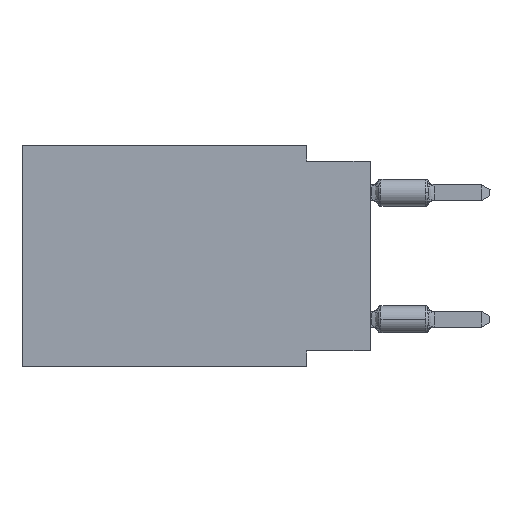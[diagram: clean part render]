
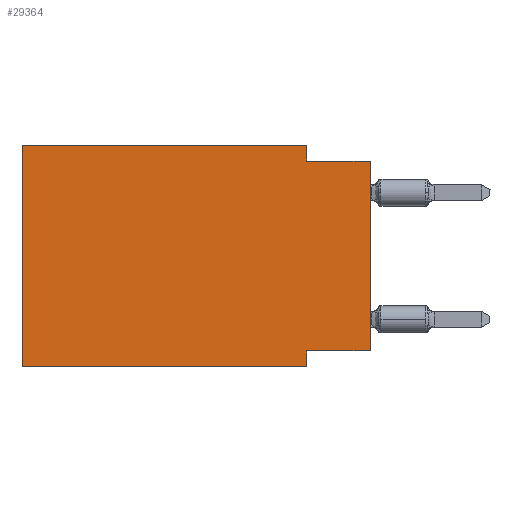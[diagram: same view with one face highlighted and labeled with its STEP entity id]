
A CAD part, left-side view. The second image highlights one B-rep face of the part: STEP entity #29364.
In plain terms, the highlighted planar face has unit normal (-1, 0, 0).
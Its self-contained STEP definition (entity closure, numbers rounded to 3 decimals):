
#2021 = DIRECTION ( 'NONE',  ( 0., -1., 0. ) ) ;
#2461 = CARTESIAN_POINT ( 'NONE',  ( 0., 0., -0.635 ) ) ;
#3961 = LINE ( 'NONE', #53313, #49097 ) ;
#5536 = DIRECTION ( 'NONE',  ( 0., 1., 0. ) ) ;
#6304 = CARTESIAN_POINT ( 'NONE',  ( 0., 13.97, 0. ) ) ;
#8507 = CARTESIAN_POINT ( 'NONE',  ( 0., 0., -8.255 ) ) ;
#9476 = CARTESIAN_POINT ( 'NONE',  ( 0., 0., -8.255 ) ) ;
#12261 = VERTEX_POINT ( 'NONE', #36278 ) ;
#12854 = LINE ( 'NONE', #33923, #29108 ) ;
#14314 = CARTESIAN_POINT ( 'NONE',  ( 0., 13.97, -8.89 ) ) ;
#15795 = ORIENTED_EDGE ( 'NONE', *, *, #59876, .F. ) ;
#16778 = VERTEX_POINT ( 'NONE', #42042 ) ;
#18086 = CARTESIAN_POINT ( 'NONE',  ( 0., 2.54, 0. ) ) ;
#18163 = EDGE_CURVE ( 'NONE', #12261, #36258, #45525, .T. ) ;
#18897 = DIRECTION ( 'NONE',  ( 0., 0., -1. ) ) ;
#21509 = CARTESIAN_POINT ( 'NONE',  ( 0., 0., -0.635 ) ) ;
#22657 = ORIENTED_EDGE ( 'NONE', *, *, #27239, .F. ) ;
#24183 = DIRECTION ( 'NONE',  ( 1., 0., 0. ) ) ;
#25414 = VECTOR ( 'NONE', #57253, 1000. ) ;
#25524 = VECTOR ( 'NONE', #40719, 1000. ) ;
#25767 = EDGE_LOOP ( 'NONE', ( #29877, #28034, #40921, #15795, #50208, #28867, #22657, #38888 ) ) ;
#27239 = EDGE_CURVE ( 'NONE', #38077, #16778, #3961, .T. ) ;
#27383 = LINE ( 'NONE', #27701, #25414 ) ;
#27456 = VERTEX_POINT ( 'NONE', #14314 ) ;
#27701 = CARTESIAN_POINT ( 'NONE',  ( 0., 13.97, -8.89 ) ) ;
#28034 = ORIENTED_EDGE ( 'NONE', *, *, #18163, .F. ) ;
#28680 = VERTEX_POINT ( 'NONE', #43931 ) ;
#28867 = ORIENTED_EDGE ( 'NONE', *, *, #59912, .T. ) ;
#29108 = VECTOR ( 'NONE', #33284, 1000. ) ;
#29364 = ADVANCED_FACE ( 'NONE', ( #64038 ), #59511, .F. ) ;
#29877 = ORIENTED_EDGE ( 'NONE', *, *, #52129, .T. ) ;
#33284 = DIRECTION ( 'NONE',  ( 0., 0., -1. ) ) ;
#33923 = CARTESIAN_POINT ( 'NONE',  ( 0., 2.54, 0. ) ) ;
#34381 = VECTOR ( 'NONE', #2021, 1000. ) ;
#35752 = DIRECTION ( 'NONE',  ( 0., 0., 1. ) ) ;
#35804 = VECTOR ( 'NONE', #60803, 1000. ) ;
#36258 = VERTEX_POINT ( 'NONE', #2461 ) ;
#36278 = CARTESIAN_POINT ( 'NONE',  ( 0., 2.54, -0.635 ) ) ;
#36370 = CARTESIAN_POINT ( 'NONE',  ( 0., 0., 0. ) ) ;
#38077 = VERTEX_POINT ( 'NONE', #58702 ) ;
#38294 = VERTEX_POINT ( 'NONE', #18086 ) ;
#38804 = DIRECTION ( 'NONE',  ( 0., 0., -1. ) ) ;
#38888 = ORIENTED_EDGE ( 'NONE', *, *, #45697, .F. ) ;
#38896 = EDGE_CURVE ( 'NONE', #27456, #28680, #60504, .T. ) ;
#40719 = DIRECTION ( 'NONE',  ( 0., 0., 1. ) ) ;
#40921 = ORIENTED_EDGE ( 'NONE', *, *, #47215, .F. ) ;
#41686 = VECTOR ( 'NONE', #5536, 1000. ) ;
#42042 = CARTESIAN_POINT ( 'NONE',  ( 0., 2.54, -8.89 ) ) ;
#43931 = CARTESIAN_POINT ( 'NONE',  ( 0., 13.97, 0. ) ) ;
#44278 = CARTESIAN_POINT ( 'NONE',  ( 0., 13.97, 0. ) ) ;
#44645 = VECTOR ( 'NONE', #35752, 1000. ) ;
#45525 = LINE ( 'NONE', #21509, #34381 ) ;
#45697 = EDGE_CURVE ( 'NONE', #55185, #38077, #54858, .T. ) ;
#47215 = EDGE_CURVE ( 'NONE', #38294, #12261, #12854, .T. ) ;
#49097 = VECTOR ( 'NONE', #18897, 1000. ) ;
#49463 = AXIS2_PLACEMENT_3D ( 'NONE', #44278, #24183, #38804 ) ;
#50208 = ORIENTED_EDGE ( 'NONE', *, *, #38896, .F. ) ;
#52129 = EDGE_CURVE ( 'NONE', #55185, #36258, #55211, .T. ) ;
#53313 = CARTESIAN_POINT ( 'NONE',  ( 0., 2.54, -8.89 ) ) ;
#54858 = LINE ( 'NONE', #9476, #41686 ) ;
#54982 = LINE ( 'NONE', #6304, #35804 ) ;
#55185 = VERTEX_POINT ( 'NONE', #8507 ) ;
#55211 = LINE ( 'NONE', #36370, #44645 ) ;
#57253 = DIRECTION ( 'NONE',  ( 0., -1., 0. ) ) ;
#58702 = CARTESIAN_POINT ( 'NONE',  ( 0., 2.54, -8.255 ) ) ;
#59511 = PLANE ( 'NONE',  #49463 ) ;
#59876 = EDGE_CURVE ( 'NONE', #28680, #38294, #54982, .T. ) ;
#59912 = EDGE_CURVE ( 'NONE', #27456, #16778, #27383, .T. ) ;
#60504 = LINE ( 'NONE', #61460, #25524 ) ;
#60803 = DIRECTION ( 'NONE',  ( 0., -1., 0. ) ) ;
#61460 = CARTESIAN_POINT ( 'NONE',  ( 0., 13.97, 0. ) ) ;
#64038 = FACE_OUTER_BOUND ( 'NONE', #25767, .T. ) ;
